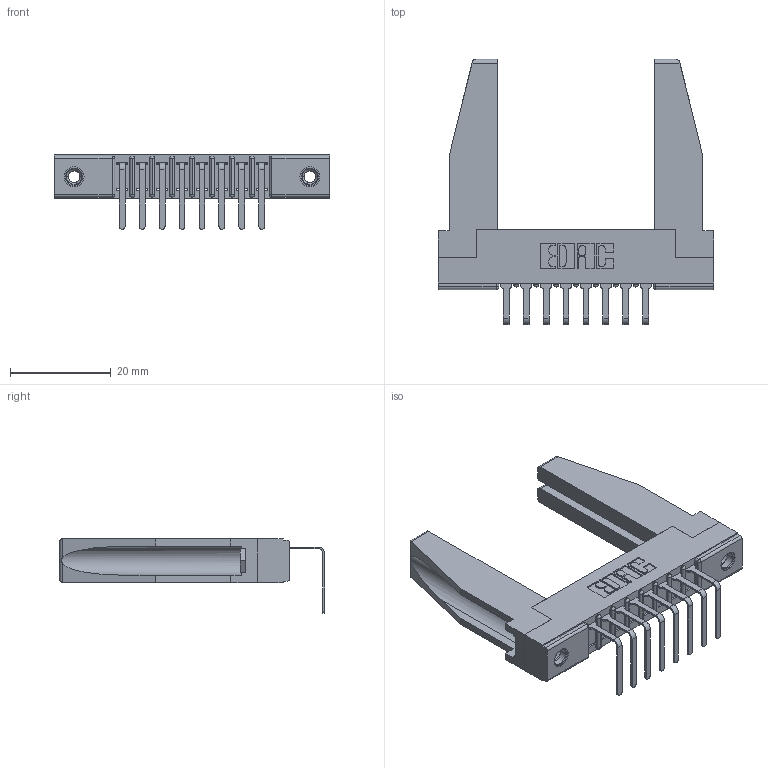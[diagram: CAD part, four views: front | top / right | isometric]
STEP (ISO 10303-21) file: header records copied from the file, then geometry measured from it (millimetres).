
FILE_DESCRIPTION (( 'STEP AP203' ), '1' );
FILE_NAME ('307-008-558-178.STEP', '2019-09-04T12:01:35', ( '' ), ( '' ), 'SwSTEP 2.0', 'SolidWorks 2016', '' );
FILE_SCHEMA (( 'CONFIG_CONTROL_DESIGN' ));
Length unit declared in the file: inch
Products named in the file (5): 307 Part_.156 Dia Mounting Holes; 307-008-558-178; 345-250-001_345-250-001-102; 307-220-078; 307-290-001_558 - 2 (Single)
Assembly tree (13 placements, depth 2):
  307-008-558-178
    307 Part_.156 Dia Mounting Holes
    307-290-001_558 - 2 (Single)  x8
    307-220-078  x2
    345-250-001_345-250-001-102  x2
Bounding box: 54.71 x 52.67 x 14.81 mm (x, y, z)
Volume: 7518.8 mm3; surface area: 8988.2 mm2
Topology: 13 solids, 13 shells, 737 faces, 2045 edges, 1318 vertices
Faces by surface type: plane 466, cylinder 237, sphere 18, cone 12, torus 4
Entity records: 13593 total; most frequent: CARTESIAN_POINT 2278, ORIENTED_EDGE 2220, DIRECTION 2192, EDGE_CURVE 1110, LINE 840, VECTOR 840, VERTEX_POINT 720, AXIS2_PLACEMENT_3D 676
